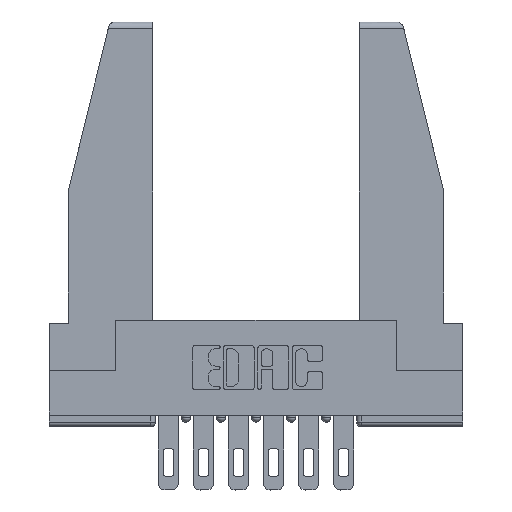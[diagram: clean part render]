
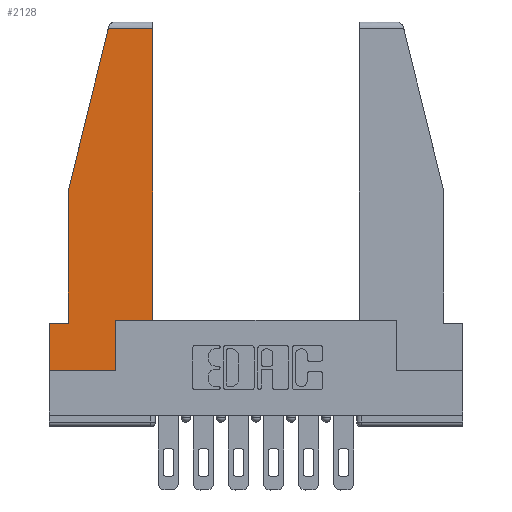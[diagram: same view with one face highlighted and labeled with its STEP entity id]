
A CAD part, top view. The second image highlights one B-rep face of the part: STEP entity #2128.
In plain terms, the highlighted planar face has unit normal (0, 0, 1).
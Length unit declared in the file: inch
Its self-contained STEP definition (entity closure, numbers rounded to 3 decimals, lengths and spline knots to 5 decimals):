
#350 = EDGE_CURVE ( 'NONE', #9865, #735, #10031, .T. ) ;
#407 = CARTESIAN_POINT ( 'NONE',  ( 0., 0.21, 0. ) ) ;
#521 = VECTOR ( 'NONE', #11730, 39.37008 ) ;
#548 = VECTOR ( 'NONE', #2244, 39.37008 ) ;
#621 = EDGE_CURVE ( 'NONE', #4001, #8296, #7659, .T. ) ;
#735 = VERTEX_POINT ( 'NONE', #2205 ) ;
#834 = LINE ( 'NONE', #10864, #548 ) ;
#1142 = VERTEX_POINT ( 'NONE', #9216 ) ;
#1697 = DIRECTION ( 'NONE',  ( 0., 1., 0. ) ) ;
#1811 = PLANE ( 'NONE',  #4520 ) ;
#1944 = CARTESIAN_POINT ( 'NONE',  ( 0.2636, 1.52, 0. ) ) ;
#2051 = DIRECTION ( 'NONE',  ( 0., -1., 0. ) ) ;
#2095 = EDGE_CURVE ( 'NONE', #735, #2190, #7770, .T. ) ;
#2128 = ADVANCED_FACE ( 'NONE', ( #11750 ), #1811, .T. ) ;
#2136 = LINE ( 'NONE', #8961, #4801 ) ;
#2190 = VERTEX_POINT ( 'NONE', #12130 ) ;
#2205 = CARTESIAN_POINT ( 'NONE',  ( 0.461, 0.223, 0. ) ) ;
#2235 = ORIENTED_EDGE ( 'NONE', *, *, #7219, .T. ) ;
#2244 = DIRECTION ( 'NONE',  ( -1., 0., 0. ) ) ;
#2268 = LINE ( 'NONE', #6155, #521 ) ;
#2576 = CARTESIAN_POINT ( 'NONE',  ( 0.297, 0.223, 0. ) ) ;
#2899 = ORIENTED_EDGE ( 'NONE', *, *, #9858, .T. ) ;
#2908 = EDGE_CURVE ( 'NONE', #11851, #4197, #2268, .T. ) ;
#3234 = ORIENTED_EDGE ( 'NONE', *, *, #9232, .T. ) ;
#3773 = LINE ( 'NONE', #7238, #8650 ) ;
#3967 = VECTOR ( 'NONE', #1697, 39.37008 ) ;
#4001 = VERTEX_POINT ( 'NONE', #407 ) ;
#4197 = VERTEX_POINT ( 'NONE', #5470 ) ;
#4520 = AXIS2_PLACEMENT_3D ( 'NONE', #4627, #6343, #7438 ) ;
#4524 = VECTOR ( 'NONE', #11179, 39.37008 ) ;
#4614 = CARTESIAN_POINT ( 'NONE',  ( 0.086, 0.8, 0. ) ) ;
#4627 = CARTESIAN_POINT ( 'NONE',  ( 0., 0., 0. ) ) ;
#4642 = ORIENTED_EDGE ( 'NONE', *, *, #9159, .T. ) ;
#4720 = ORIENTED_EDGE ( 'NONE', *, *, #2095, .T. ) ;
#4801 = VECTOR ( 'NONE', #9909, 39.37008 ) ;
#4858 = CARTESIAN_POINT ( 'NONE',  ( 0., 0.21, 0. ) ) ;
#4975 = ORIENTED_EDGE ( 'NONE', *, *, #2908, .T. ) ;
#5115 = ORIENTED_EDGE ( 'NONE', *, *, #6513, .T. ) ;
#5132 = ORIENTED_EDGE ( 'NONE', *, *, #350, .T. ) ;
#5442 = VECTOR ( 'NONE', #8278, 39.37008 ) ;
#5470 = CARTESIAN_POINT ( 'NONE',  ( 0.086, 0.8, 0. ) ) ;
#6155 = CARTESIAN_POINT ( 'NONE',  ( 0.271, 1.55, 0. ) ) ;
#6343 = DIRECTION ( 'NONE',  ( 0., 0., 1. ) ) ;
#6513 = EDGE_CURVE ( 'NONE', #4197, #9256, #11950, .T. ) ;
#7165 = DIRECTION ( 'NONE',  ( -1., 0., 0. ) ) ;
#7219 = EDGE_CURVE ( 'NONE', #1142, #9865, #8709, .T. ) ;
#7238 = CARTESIAN_POINT ( 'NONE',  ( 0., 1.52, 0. ) ) ;
#7438 = DIRECTION ( 'NONE',  ( 1., 0., 0. ) ) ;
#7659 = LINE ( 'NONE', #4858, #9724 ) ;
#7770 = LINE ( 'NONE', #9083, #4524 ) ;
#8258 = VECTOR ( 'NONE', #10113, 39.37008 ) ;
#8278 = DIRECTION ( 'NONE',  ( 1., 0., 0. ) ) ;
#8296 = VERTEX_POINT ( 'NONE', #10067 ) ;
#8650 = VECTOR ( 'NONE', #7165, 39.37008 ) ;
#8709 = LINE ( 'NONE', #11190, #3967 ) ;
#8961 = CARTESIAN_POINT ( 'NONE',  ( 0., 0., 0. ) ) ;
#9083 = CARTESIAN_POINT ( 'NONE',  ( 0.461, 0.223, 0. ) ) ;
#9159 = EDGE_CURVE ( 'NONE', #9256, #4001, #834, .T. ) ;
#9216 = CARTESIAN_POINT ( 'NONE',  ( 0.297, 0., 0. ) ) ;
#9232 = EDGE_CURVE ( 'NONE', #2190, #11851, #3773, .T. ) ;
#9256 = VERTEX_POINT ( 'NONE', #10009 ) ;
#9308 = ORIENTED_EDGE ( 'NONE', *, *, #621, .T. ) ;
#9724 = VECTOR ( 'NONE', #2051, 39.37008 ) ;
#9858 = EDGE_CURVE ( 'NONE', #8296, #1142, #2136, .T. ) ;
#9865 = VERTEX_POINT ( 'NONE', #10850 ) ;
#9909 = DIRECTION ( 'NONE',  ( 1., 0., 0. ) ) ;
#10009 = CARTESIAN_POINT ( 'NONE',  ( 0.086, 0.21, 0. ) ) ;
#10031 = LINE ( 'NONE', #2576, #5442 ) ;
#10067 = CARTESIAN_POINT ( 'NONE',  ( 0., 0., 0. ) ) ;
#10113 = DIRECTION ( 'NONE',  ( 0., -1., 0. ) ) ;
#10832 = EDGE_LOOP ( 'NONE', ( #4720, #3234, #4975, #5115, #4642, #9308, #2899, #2235, #5132 ) ) ;
#10850 = CARTESIAN_POINT ( 'NONE',  ( 0.297, 0.223, 0. ) ) ;
#10864 = CARTESIAN_POINT ( 'NONE',  ( 0., 0.21, 0. ) ) ;
#11179 = DIRECTION ( 'NONE',  ( 0., 1., 0. ) ) ;
#11190 = CARTESIAN_POINT ( 'NONE',  ( 0.297, 0., 0. ) ) ;
#11730 = DIRECTION ( 'NONE',  ( -0.239, -0.971, 0. ) ) ;
#11750 = FACE_OUTER_BOUND ( 'NONE', #10832, .T. ) ;
#11851 = VERTEX_POINT ( 'NONE', #1944 ) ;
#11950 = LINE ( 'NONE', #4614, #8258 ) ;
#12130 = CARTESIAN_POINT ( 'NONE',  ( 0.461, 1.52, 0. ) ) ;
